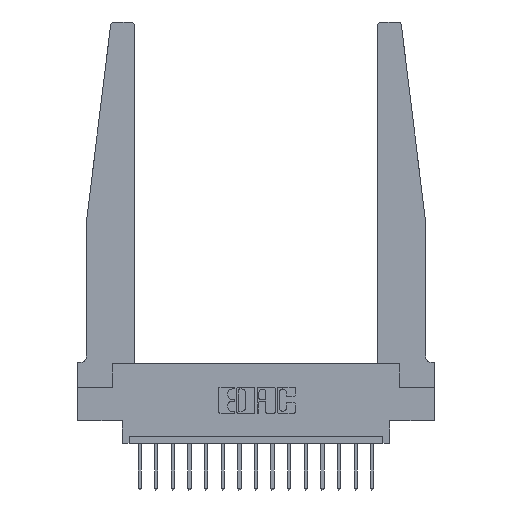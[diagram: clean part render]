
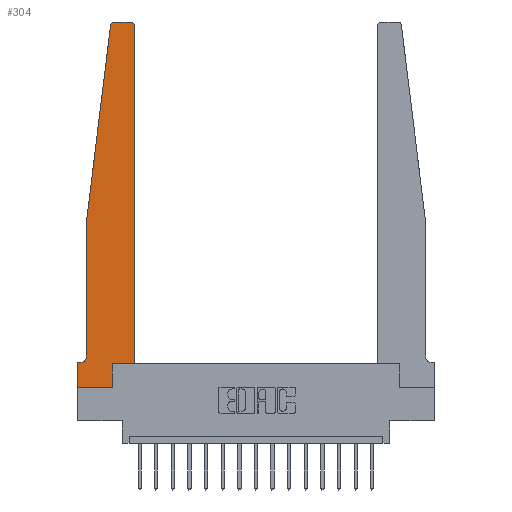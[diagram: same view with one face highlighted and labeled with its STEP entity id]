
A CAD part, top view. The second image highlights one B-rep face of the part: STEP entity #304.
In plain terms, the highlighted planar face has unit normal (0, 0, 1).
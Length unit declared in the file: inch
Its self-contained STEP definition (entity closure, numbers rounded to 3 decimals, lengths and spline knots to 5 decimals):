
#273 = LINE ( 'NONE', #15768, #10309 ) ;
#304 = ADVANCED_FACE ( 'NONE', ( #13511 ), #16373, .T. ) ;
#319 = AXIS2_PLACEMENT_3D ( 'NONE', #5410, #7129, #5674 ) ;
#365 = VERTEX_POINT ( 'NONE', #14139 ) ;
#689 = CARTESIAN_POINT ( 'NONE',  ( 0.425, 0.18, 0.37 ) ) ;
#752 = EDGE_CURVE ( 'NONE', #14404, #1333, #4188, .T. ) ;
#1201 = DIRECTION ( 'NONE',  ( 0., 0., -1. ) ) ;
#1306 = VECTOR ( 'NONE', #8708, 39.37008 ) ;
#1333 = VERTEX_POINT ( 'NONE', #3506 ) ;
#1377 = AXIS2_PLACEMENT_3D ( 'NONE', #8193, #1201, #6907 ) ;
#1517 = ORIENTED_EDGE ( 'NONE', *, *, #12362, .T. ) ;
#1785 = AXIS2_PLACEMENT_3D ( 'NONE', #9263, #3765, #13785 ) ;
#1811 = CARTESIAN_POINT ( 'NONE',  ( 0., 0., 0.37 ) ) ;
#2876 = DIRECTION ( 'NONE',  ( -0.122, -0.992, 0. ) ) ;
#3506 = CARTESIAN_POINT ( 'NONE',  ( 0.395, 2.75, 0.37 ) ) ;
#3546 = ORIENTED_EDGE ( 'NONE', *, *, #752, .T. ) ;
#3750 = DIRECTION ( 'NONE',  ( 0., 0., 1. ) ) ;
#3759 = VERTEX_POINT ( 'NONE', #15296 ) ;
#3765 = DIRECTION ( 'NONE',  ( 0., 0., 1. ) ) ;
#4150 = EDGE_CURVE ( 'NONE', #6568, #6464, #17731, .T. ) ;
#4188 = CIRCLE ( 'NONE', #319, 0.03 ) ;
#4616 = LINE ( 'NONE', #7346, #16937 ) ;
#4820 = DIRECTION ( 'NONE',  ( 0., -1., 0. ) ) ;
#4905 = CARTESIAN_POINT ( 'NONE',  ( 0., 0.1875, 0.37 ) ) ;
#5040 = VERTEX_POINT ( 'NONE', #15668 ) ;
#5231 = CARTESIAN_POINT ( 'NONE',  ( 0.27653, 2.72, 0.37 ) ) ;
#5410 = CARTESIAN_POINT ( 'NONE',  ( 0.395, 2.72, 0.37 ) ) ;
#5674 = DIRECTION ( 'NONE',  ( 1., 0., 0. ) ) ;
#5753 = CARTESIAN_POINT ( 'NONE',  ( 0.425, 2.72, 0.37 ) ) ;
#5895 = LINE ( 'NONE', #9000, #7327 ) ;
#6031 = EDGE_CURVE ( 'NONE', #9872, #18292, #273, .T. ) ;
#6206 = CARTESIAN_POINT ( 'NONE',  ( 0.065, 1.25, 0.37 ) ) ;
#6337 = DIRECTION ( 'NONE',  ( 1., 0., 0. ) ) ;
#6464 = VERTEX_POINT ( 'NONE', #12616 ) ;
#6568 = VERTEX_POINT ( 'NONE', #4905 ) ;
#6614 = ORIENTED_EDGE ( 'NONE', *, *, #9038, .T. ) ;
#6805 = CARTESIAN_POINT ( 'NONE',  ( 0.24675, 2.72367, 0.37 ) ) ;
#6907 = DIRECTION ( 'NONE',  ( -1., 0., 0. ) ) ;
#6995 = EDGE_CURVE ( 'NONE', #365, #12502, #5895, .T. ) ;
#7015 = EDGE_CURVE ( 'NONE', #12502, #14404, #15816, .T. ) ;
#7089 = DIRECTION ( 'NONE',  ( -1., 0., 0. ) ) ;
#7129 = DIRECTION ( 'NONE',  ( 0., 0., 1. ) ) ;
#7258 = DIRECTION ( 'NONE',  ( 0., 1., 0. ) ) ;
#7327 = VECTOR ( 'NONE', #11681, 39.37008 ) ;
#7339 = CARTESIAN_POINT ( 'NONE',  ( 0.425, 0.18, 0.37 ) ) ;
#7346 = CARTESIAN_POINT ( 'NONE',  ( 0.065, 0.1875, 0.37 ) ) ;
#7532 = DIRECTION ( 'NONE',  ( -1., 0., 0. ) ) ;
#7880 = ORIENTED_EDGE ( 'NONE', *, *, #9857, .T. ) ;
#8077 = EDGE_CURVE ( 'NONE', #18292, #9935, #10119, .T. ) ;
#8193 = CARTESIAN_POINT ( 'NONE',  ( 0.015, 0.2375, 0.37 ) ) ;
#8228 = ORIENTED_EDGE ( 'NONE', *, *, #10886, .T. ) ;
#8689 = CARTESIAN_POINT ( 'NONE',  ( 0.065, 1.25, 0.37 ) ) ;
#8708 = DIRECTION ( 'NONE',  ( 1., 0., 0. ) ) ;
#9000 = CARTESIAN_POINT ( 'NONE',  ( 0.425, 0.18, 0.37 ) ) ;
#9038 = EDGE_CURVE ( 'NONE', #10986, #9872, #11015, .T. ) ;
#9153 = ORIENTED_EDGE ( 'NONE', *, *, #4150, .T. ) ;
#9263 = CARTESIAN_POINT ( 'NONE',  ( 0., 0.1875, 0.37 ) ) ;
#9434 = ORIENTED_EDGE ( 'NONE', *, *, #16236, .T. ) ;
#9485 = ORIENTED_EDGE ( 'NONE', *, *, #6995, .T. ) ;
#9505 = ORIENTED_EDGE ( 'NONE', *, *, #6031, .T. ) ;
#9857 = EDGE_CURVE ( 'NONE', #3759, #365, #15539, .T. ) ;
#9872 = VERTEX_POINT ( 'NONE', #6805 ) ;
#9935 = VERTEX_POINT ( 'NONE', #12416 ) ;
#10119 = LINE ( 'NONE', #6206, #18057 ) ;
#10309 = VECTOR ( 'NONE', #2876, 39.37008 ) ;
#10417 = AXIS2_PLACEMENT_3D ( 'NONE', #5231, #3750, #6337 ) ;
#10495 = CARTESIAN_POINT ( 'NONE',  ( 0., 0., 0.37 ) ) ;
#10788 = ORIENTED_EDGE ( 'NONE', *, *, #8077, .T. ) ;
#10886 = EDGE_CURVE ( 'NONE', #5040, #6568, #4616, .T. ) ;
#10986 = VERTEX_POINT ( 'NONE', #16009 ) ;
#11015 = CIRCLE ( 'NONE', #10417, 0.03 ) ;
#11496 = LINE ( 'NONE', #17133, #17846 ) ;
#11681 = DIRECTION ( 'NONE',  ( 1., 0., 0. ) ) ;
#11735 = VECTOR ( 'NONE', #11979, 39.37008 ) ;
#11979 = DIRECTION ( 'NONE',  ( 0., -1., 0. ) ) ;
#12230 = VECTOR ( 'NONE', #15439, 39.37008 ) ;
#12362 = EDGE_CURVE ( 'NONE', #6464, #3759, #17115, .T. ) ;
#12416 = CARTESIAN_POINT ( 'NONE',  ( 0.065, 0.2375, 0.37 ) ) ;
#12502 = VERTEX_POINT ( 'NONE', #689 ) ;
#12616 = CARTESIAN_POINT ( 'NONE',  ( 0., 0., 0.37 ) ) ;
#13511 = FACE_OUTER_BOUND ( 'NONE', #15953, .T. ) ;
#13785 = DIRECTION ( 'NONE',  ( 1., 0., 0. ) ) ;
#13793 = CARTESIAN_POINT ( 'NONE',  ( 0.2605, 0.18, 0.37 ) ) ;
#13915 = ORIENTED_EDGE ( 'NONE', *, *, #7015, .T. ) ;
#14139 = CARTESIAN_POINT ( 'NONE',  ( 0.2605, 0.18, 0.37 ) ) ;
#14404 = VERTEX_POINT ( 'NONE', #5753 ) ;
#15296 = CARTESIAN_POINT ( 'NONE',  ( 0.2605, 0., 0.37 ) ) ;
#15439 = DIRECTION ( 'NONE',  ( 0., 1., 0. ) ) ;
#15539 = LINE ( 'NONE', #13793, #12230 ) ;
#15609 = ORIENTED_EDGE ( 'NONE', *, *, #17243, .T. ) ;
#15668 = CARTESIAN_POINT ( 'NONE',  ( 0.015, 0.1875, 0.37 ) ) ;
#15768 = CARTESIAN_POINT ( 'NONE',  ( 0.065, 1.25, 0.37 ) ) ;
#15777 = CIRCLE ( 'NONE', #1377, 0.05 ) ;
#15816 = LINE ( 'NONE', #7339, #17967 ) ;
#15953 = EDGE_LOOP ( 'NONE', ( #9434, #6614, #9505, #10788, #15609, #8228, #9153, #1517, #7880, #9485, #13915, #3546 ) ) ;
#16009 = CARTESIAN_POINT ( 'NONE',  ( 0.27653, 2.75, 0.37 ) ) ;
#16236 = EDGE_CURVE ( 'NONE', #1333, #10986, #11496, .T. ) ;
#16373 = PLANE ( 'NONE',  #1785 ) ;
#16937 = VECTOR ( 'NONE', #7532, 39.37008 ) ;
#17115 = LINE ( 'NONE', #1811, #1306 ) ;
#17133 = CARTESIAN_POINT ( 'NONE',  ( 0.25, 2.75, 0.37 ) ) ;
#17243 = EDGE_CURVE ( 'NONE', #9935, #5040, #15777, .T. ) ;
#17731 = LINE ( 'NONE', #10495, #11735 ) ;
#17846 = VECTOR ( 'NONE', #7089, 39.37008 ) ;
#17967 = VECTOR ( 'NONE', #7258, 39.37008 ) ;
#18057 = VECTOR ( 'NONE', #4820, 39.37008 ) ;
#18292 = VERTEX_POINT ( 'NONE', #8689 ) ;
